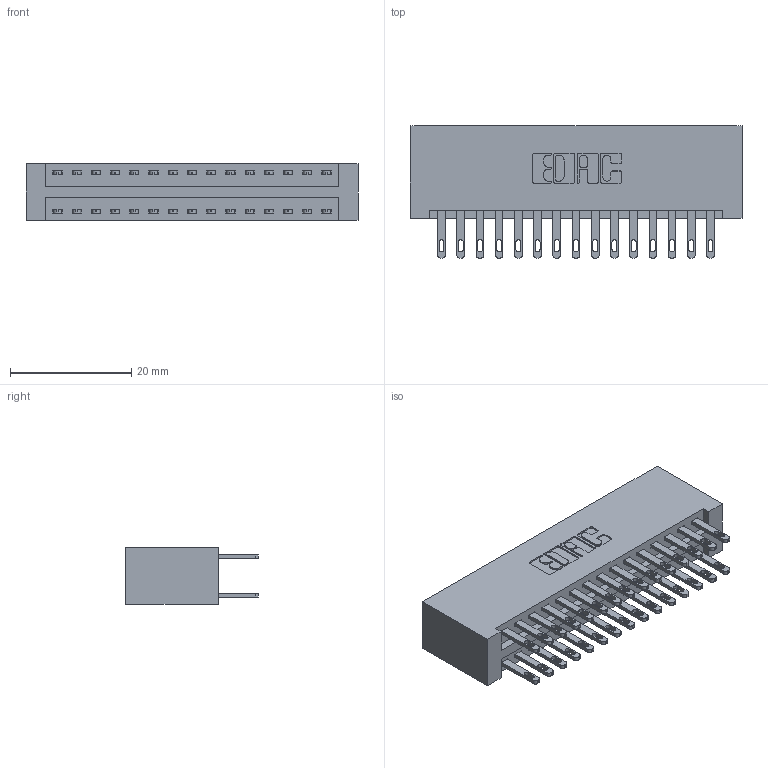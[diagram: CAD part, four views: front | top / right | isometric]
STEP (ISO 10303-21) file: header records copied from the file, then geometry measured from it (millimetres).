
FILE_DESCRIPTION (( 'STEP AP203' ), '1' );
FILE_NAME ('346-030-500-201.STEP', '2018-08-22T03:57:20', ( '' ), ( '' ), 'SwSTEP 2.0', 'SolidWorks 2016', '' );
FILE_SCHEMA (( 'CONFIG_CONTROL_DESIGN' ));
Length unit declared in the file: inch
Products named in the file (3): 346 Part_No Mounting Lugs; 345-292-001_345-293-100; 346-030-500-201
Assembly tree (31 placements, depth 2):
  346-030-500-201
    346 Part_No Mounting Lugs
    345-292-001_345-293-100  x30
Bounding box: 54.86 x 21.84 x 9.4 mm (x, y, z)
Volume: 5805.2 mm3; surface area: 8032.4 mm2
Topology: 31 solids, 31 shells, 1554 faces, 4715 edges, 3142 vertices
Faces by surface type: plane 942, cylinder 612
Entity records: 13077 total; most frequent: CARTESIAN_POINT 2188, ORIENTED_EDGE 2122, DIRECTION 1977, EDGE_CURVE 1061, LINE 873, VECTOR 873, VERTEX_POINT 706, AXIS2_PLACEMENT_3D 552
